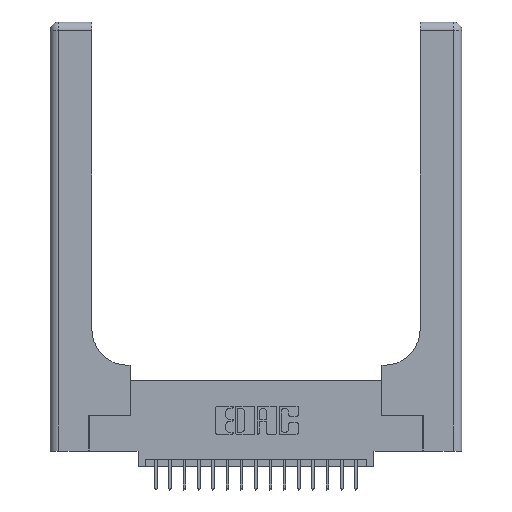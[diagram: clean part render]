
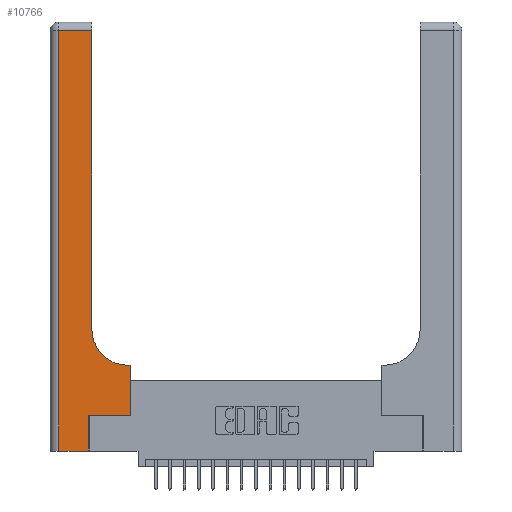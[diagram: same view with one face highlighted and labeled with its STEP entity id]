
A CAD part, top view. The second image highlights one B-rep face of the part: STEP entity #10766.
In plain terms, the highlighted planar face has unit normal (0, 0, 1).
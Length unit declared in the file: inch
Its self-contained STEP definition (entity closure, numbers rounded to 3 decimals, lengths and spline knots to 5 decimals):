
#41 = CARTESIAN_POINT ( 'NONE',  ( 0.5585, 0.25, 0.37 ) ) ;
#62 = ORIENTED_EDGE ( 'NONE', *, *, #20813, .T. ) ;
#336 = CARTESIAN_POINT ( 'NONE',  ( 0.06, 3., 0.37 ) ) ;
#469 = ORIENTED_EDGE ( 'NONE', *, *, #11472, .T. ) ;
#1122 = CARTESIAN_POINT ( 'NONE',  ( 0., 2.94, 0.37 ) ) ;
#1136 = VERTEX_POINT ( 'NONE', #11657 ) ;
#1256 = CARTESIAN_POINT ( 'NONE',  ( 0.269, 0., 0.37 ) ) ;
#1594 = LINE ( 'NONE', #1122, #16140 ) ;
#1658 = DIRECTION ( 'NONE',  ( 0., 1., 0. ) ) ;
#3010 = CARTESIAN_POINT ( 'NONE',  ( 0.5585, 0.6, 0.37 ) ) ;
#3599 = CARTESIAN_POINT ( 'NONE',  ( 0.269, 0., 0.37 ) ) ;
#3726 = EDGE_CURVE ( 'NONE', #1136, #10802, #13951, .T. ) ;
#3727 = EDGE_CURVE ( 'NONE', #12051, #20289, #16932, .T. ) ;
#4477 = VERTEX_POINT ( 'NONE', #9543 ) ;
#4519 = CARTESIAN_POINT ( 'NONE',  ( 0.269, 0.25, 0.37 ) ) ;
#4912 = LINE ( 'NONE', #14533, #16964 ) ;
#5062 = EDGE_LOOP ( 'NONE', ( #20546, #62, #12669, #469, #7148, #14362, #18632, #7745, #8470 ) ) ;
#5101 = CARTESIAN_POINT ( 'NONE',  ( 0.269, 0.25, 0.37 ) ) ;
#5847 = VERTEX_POINT ( 'NONE', #3599 ) ;
#6329 = PLANE ( 'NONE',  #7435 ) ;
#6472 = VERTEX_POINT ( 'NONE', #14908 ) ;
#6520 = DIRECTION ( 'NONE',  ( -1., 0., 0. ) ) ;
#7148 = ORIENTED_EDGE ( 'NONE', *, *, #14388, .T. ) ;
#7435 = AXIS2_PLACEMENT_3D ( 'NONE', #8438, #8367, #19615 ) ;
#7650 = DIRECTION ( 'NONE',  ( 0., 1., 0. ) ) ;
#7745 = ORIENTED_EDGE ( 'NONE', *, *, #14759, .T. ) ;
#8000 = LINE ( 'NONE', #336, #12576 ) ;
#8367 = DIRECTION ( 'NONE',  ( 0., 0., -1. ) ) ;
#8438 = CARTESIAN_POINT ( 'NONE',  ( 0., 3., 0.37 ) ) ;
#8470 = ORIENTED_EDGE ( 'NONE', *, *, #11729, .T. ) ;
#8471 = DIRECTION ( 'NONE',  ( 0., -1., 0. ) ) ;
#8745 = CARTESIAN_POINT ( 'NONE',  ( 0., 0., 0.37 ) ) ;
#8776 = AXIS2_PLACEMENT_3D ( 'NONE', #9099, #20414, #12337 ) ;
#9099 = CARTESIAN_POINT ( 'NONE',  ( 0.5415, 0.85, 0.37 ) ) ;
#9543 = CARTESIAN_POINT ( 'NONE',  ( 0.06, 2.94, 0.37 ) ) ;
#9856 = VECTOR ( 'NONE', #16591, 39.37008 ) ;
#10627 = FACE_OUTER_BOUND ( 'NONE', #5062, .T. ) ;
#10766 = ADVANCED_FACE ( 'NONE', ( #10627 ), #6329, .F. ) ;
#10802 = VERTEX_POINT ( 'NONE', #19686 ) ;
#11472 = EDGE_CURVE ( 'NONE', #6472, #5847, #17635, .T. ) ;
#11501 = VECTOR ( 'NONE', #7650, 39.37008 ) ;
#11657 = CARTESIAN_POINT ( 'NONE',  ( 0.2915, 0.85, 0.37 ) ) ;
#11729 = EDGE_CURVE ( 'NONE', #14620, #1136, #11853, .T. ) ;
#11853 = CIRCLE ( 'NONE', #8776, 0.25 ) ;
#12051 = VERTEX_POINT ( 'NONE', #19560 ) ;
#12125 = DIRECTION ( 'NONE',  ( 1., 0., 0. ) ) ;
#12337 = DIRECTION ( 'NONE',  ( 1., 0., 0. ) ) ;
#12576 = VECTOR ( 'NONE', #8471, 39.37008 ) ;
#12669 = ORIENTED_EDGE ( 'NONE', *, *, #13208, .T. ) ;
#12778 = LINE ( 'NONE', #4519, #13050 ) ;
#13050 = VECTOR ( 'NONE', #12125, 39.37008 ) ;
#13208 = EDGE_CURVE ( 'NONE', #4477, #6472, #8000, .T. ) ;
#13508 = EDGE_CURVE ( 'NONE', #16732, #12051, #12778, .T. ) ;
#13696 = VECTOR ( 'NONE', #14506, 39.37008 ) ;
#13951 = LINE ( 'NONE', #20757, #14454 ) ;
#14362 = ORIENTED_EDGE ( 'NONE', *, *, #13508, .T. ) ;
#14388 = EDGE_CURVE ( 'NONE', #5847, #16732, #18011, .T. ) ;
#14454 = VECTOR ( 'NONE', #1658, 39.37008 ) ;
#14506 = DIRECTION ( 'NONE',  ( 0., 1., 0. ) ) ;
#14533 = CARTESIAN_POINT ( 'NONE',  ( 0.2915, 0.6, 0.37 ) ) ;
#14620 = VERTEX_POINT ( 'NONE', #16329 ) ;
#14759 = EDGE_CURVE ( 'NONE', #20289, #14620, #4912, .T. ) ;
#14908 = CARTESIAN_POINT ( 'NONE',  ( 0.06, 0., 0.37 ) ) ;
#16140 = VECTOR ( 'NONE', #18615, 39.37008 ) ;
#16329 = CARTESIAN_POINT ( 'NONE',  ( 0.5415, 0.6, 0.37 ) ) ;
#16591 = DIRECTION ( 'NONE',  ( 1., 0., 0. ) ) ;
#16732 = VERTEX_POINT ( 'NONE', #5101 ) ;
#16932 = LINE ( 'NONE', #41, #13696 ) ;
#16964 = VECTOR ( 'NONE', #6520, 39.37008 ) ;
#17635 = LINE ( 'NONE', #8745, #9856 ) ;
#18011 = LINE ( 'NONE', #1256, #11501 ) ;
#18615 = DIRECTION ( 'NONE',  ( -1., 0., 0. ) ) ;
#18632 = ORIENTED_EDGE ( 'NONE', *, *, #3727, .T. ) ;
#19560 = CARTESIAN_POINT ( 'NONE',  ( 0.5585, 0.25, 0.37 ) ) ;
#19615 = DIRECTION ( 'NONE',  ( -1., 0., 0. ) ) ;
#19686 = CARTESIAN_POINT ( 'NONE',  ( 0.2915, 2.94, 0.37 ) ) ;
#20289 = VERTEX_POINT ( 'NONE', #3010 ) ;
#20414 = DIRECTION ( 'NONE',  ( 0., 0., -1. ) ) ;
#20546 = ORIENTED_EDGE ( 'NONE', *, *, #3726, .T. ) ;
#20757 = CARTESIAN_POINT ( 'NONE',  ( 0.2915, 3., 0.37 ) ) ;
#20813 = EDGE_CURVE ( 'NONE', #10802, #4477, #1594, .T. ) ;
